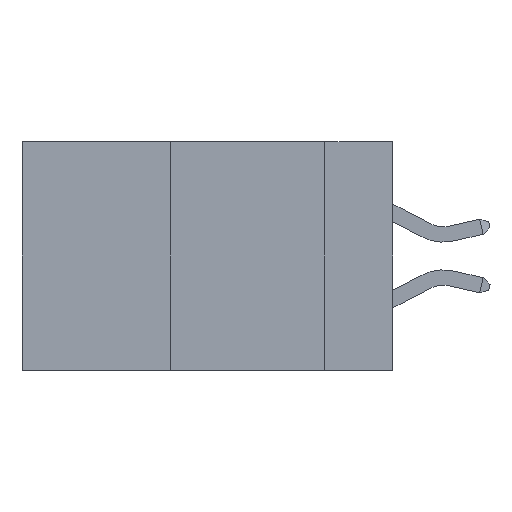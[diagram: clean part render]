
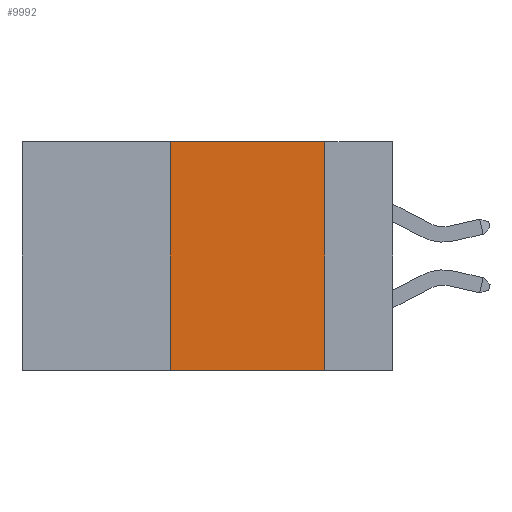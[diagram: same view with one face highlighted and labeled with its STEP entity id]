
A CAD part, left-side view. The second image highlights one B-rep face of the part: STEP entity #9992.
In plain terms, the highlighted planar face has unit normal (-1, 0, 0).
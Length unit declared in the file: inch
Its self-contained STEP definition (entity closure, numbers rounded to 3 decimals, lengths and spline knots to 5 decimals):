
#1755 = ORIENTED_EDGE ( 'NONE', *, *, #6119, .T. ) ;
#2249 = CARTESIAN_POINT ( 'NONE',  ( 0., 0.11, 0. ) ) ;
#3103 = VECTOR ( 'NONE', #28982, 39.37008 ) ;
#4367 = EDGE_CURVE ( 'NONE', #6680, #29662, #20925, .T. ) ;
#5642 = EDGE_CURVE ( 'NONE', #7333, #6680, #18345, .T. ) ;
#5902 = DIRECTION ( 'NONE',  ( 0., 0., 1. ) ) ;
#6119 = EDGE_CURVE ( 'NONE', #7333, #19766, #14970, .T. ) ;
#6680 = VERTEX_POINT ( 'NONE', #16694 ) ;
#7333 = VERTEX_POINT ( 'NONE', #17128 ) ;
#8387 = VECTOR ( 'NONE', #25579, 39.37008 ) ;
#8402 = LINE ( 'NONE', #25858, #15080 ) ;
#9992 = ADVANCED_FACE ( 'NONE', ( #13877 ), #22376, .F. ) ;
#11205 = CARTESIAN_POINT ( 'NONE',  ( 0., 0.6, -0.37 ) ) ;
#11941 = ORIENTED_EDGE ( 'NONE', *, *, #27791, .F. ) ;
#12815 = DIRECTION ( 'NONE',  ( 1., 0., 0. ) ) ;
#13877 = FACE_OUTER_BOUND ( 'NONE', #26244, .T. ) ;
#14970 = LINE ( 'NONE', #11205, #3103 ) ;
#15080 = VECTOR ( 'NONE', #18843, 39.37008 ) ;
#16694 = CARTESIAN_POINT ( 'NONE',  ( 0., 0.36, 0. ) ) ;
#17128 = CARTESIAN_POINT ( 'NONE',  ( 0., 0.36, -0.37 ) ) ;
#17359 = CARTESIAN_POINT ( 'NONE',  ( 0., 0.6, 0. ) ) ;
#17714 = CARTESIAN_POINT ( 'NONE',  ( 0., 0.36, 0. ) ) ;
#18296 = ORIENTED_EDGE ( 'NONE', *, *, #4367, .F. ) ;
#18345 = LINE ( 'NONE', #17714, #24571 ) ;
#18366 = CARTESIAN_POINT ( 'NONE',  ( 0., 0.6, 0. ) ) ;
#18843 = DIRECTION ( 'NONE',  ( 0., 0., -1. ) ) ;
#19671 = ORIENTED_EDGE ( 'NONE', *, *, #5642, .F. ) ;
#19766 = VERTEX_POINT ( 'NONE', #21543 ) ;
#20925 = LINE ( 'NONE', #18366, #8387 ) ;
#21543 = CARTESIAN_POINT ( 'NONE',  ( 0., 0.11, -0.37 ) ) ;
#22376 = PLANE ( 'NONE',  #24043 ) ;
#24043 = AXIS2_PLACEMENT_3D ( 'NONE', #17359, #12815, #26952 ) ;
#24571 = VECTOR ( 'NONE', #5902, 39.37008 ) ;
#25579 = DIRECTION ( 'NONE',  ( 0., -1., 0. ) ) ;
#25858 = CARTESIAN_POINT ( 'NONE',  ( 0., 0.11, 0. ) ) ;
#26244 = EDGE_LOOP ( 'NONE', ( #11941, #18296, #19671, #1755 ) ) ;
#26952 = DIRECTION ( 'NONE',  ( 0., 0., -1. ) ) ;
#27791 = EDGE_CURVE ( 'NONE', #29662, #19766, #8402, .T. ) ;
#28982 = DIRECTION ( 'NONE',  ( 0., -1., 0. ) ) ;
#29662 = VERTEX_POINT ( 'NONE', #2249 ) ;
